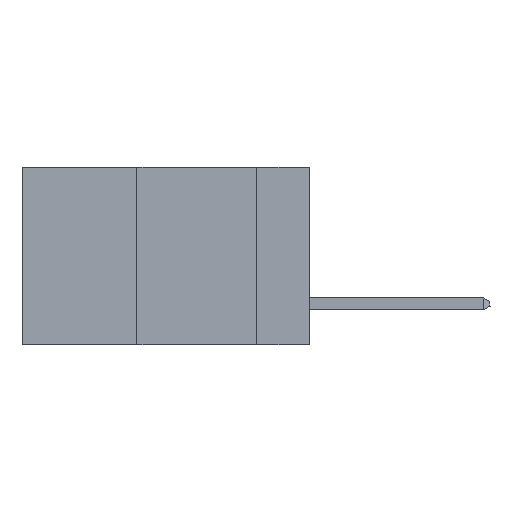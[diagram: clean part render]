
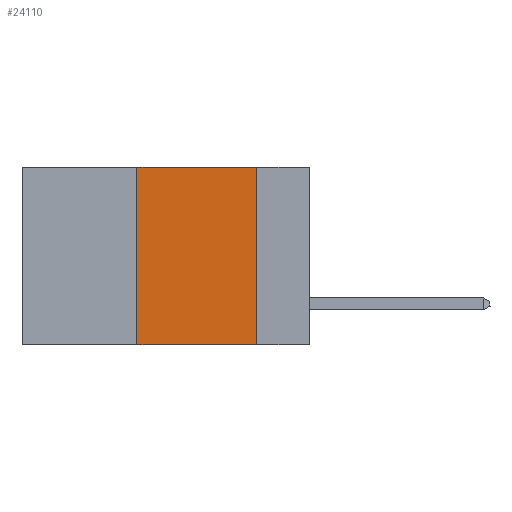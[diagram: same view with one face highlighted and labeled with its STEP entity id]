
A CAD part, left-side view. The second image highlights one B-rep face of the part: STEP entity #24110.
In plain terms, the highlighted planar face has unit normal (-1, 0, 0).
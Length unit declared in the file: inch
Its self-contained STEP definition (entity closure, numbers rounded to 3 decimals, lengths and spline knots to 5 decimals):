
#429 = CARTESIAN_POINT ( 'NONE',  ( 0., 0.6, 0. ) ) ;
#1868 = CARTESIAN_POINT ( 'NONE',  ( 0., 0.11, -0.37 ) ) ;
#2895 = DIRECTION ( 'NONE',  ( 0., 0., -1. ) ) ;
#3239 = ORIENTED_EDGE ( 'NONE', *, *, #12792, .F. ) ;
#3734 = LINE ( 'NONE', #16531, #11338 ) ;
#5599 = PLANE ( 'NONE',  #18371 ) ;
#7148 = DIRECTION ( 'NONE',  ( 0., -1., 0. ) ) ;
#7250 = CARTESIAN_POINT ( 'NONE',  ( 0., 0.11, 0. ) ) ;
#10733 = DIRECTION ( 'NONE',  ( 1., 0., 0. ) ) ;
#11338 = VECTOR ( 'NONE', #7148, 39.37008 ) ;
#11718 = VECTOR ( 'NONE', #18276, 39.37008 ) ;
#12578 = VECTOR ( 'NONE', #23292, 39.37008 ) ;
#12792 = EDGE_CURVE ( 'NONE', #22145, #31823, #23271, .T. ) ;
#13720 = LINE ( 'NONE', #25666, #12578 ) ;
#16531 = CARTESIAN_POINT ( 'NONE',  ( 0., 0.6, -0.37 ) ) ;
#16727 = EDGE_CURVE ( 'NONE', #22037, #23060, #3734, .T. ) ;
#16895 = ORIENTED_EDGE ( 'NONE', *, *, #27657, .F. ) ;
#16928 = FACE_OUTER_BOUND ( 'NONE', #29908, .T. ) ;
#18276 = DIRECTION ( 'NONE',  ( 0., -1., 0. ) ) ;
#18371 = AXIS2_PLACEMENT_3D ( 'NONE', #429, #10733, #2895 ) ;
#19839 = CARTESIAN_POINT ( 'NONE',  ( 0., 0.36, -0.37 ) ) ;
#21968 = LINE ( 'NONE', #7250, #27224 ) ;
#22037 = VERTEX_POINT ( 'NONE', #19839 ) ;
#22043 = DIRECTION ( 'NONE',  ( 0., 0., -1. ) ) ;
#22145 = VERTEX_POINT ( 'NONE', #23518 ) ;
#22545 = CARTESIAN_POINT ( 'NONE',  ( 0., 0.11, 0. ) ) ;
#23060 = VERTEX_POINT ( 'NONE', #1868 ) ;
#23271 = LINE ( 'NONE', #30961, #11718 ) ;
#23292 = DIRECTION ( 'NONE',  ( 0., 0., 1. ) ) ;
#23518 = CARTESIAN_POINT ( 'NONE',  ( 0., 0.36, 0. ) ) ;
#24110 = ADVANCED_FACE ( 'NONE', ( #16928 ), #5599, .F. ) ;
#25666 = CARTESIAN_POINT ( 'NONE',  ( 0., 0.36, 0. ) ) ;
#27224 = VECTOR ( 'NONE', #22043, 39.37008 ) ;
#27657 = EDGE_CURVE ( 'NONE', #22037, #22145, #13720, .T. ) ;
#27969 = ORIENTED_EDGE ( 'NONE', *, *, #29240, .F. ) ;
#29240 = EDGE_CURVE ( 'NONE', #31823, #23060, #21968, .T. ) ;
#29731 = ORIENTED_EDGE ( 'NONE', *, *, #16727, .T. ) ;
#29908 = EDGE_LOOP ( 'NONE', ( #27969, #3239, #16895, #29731 ) ) ;
#30961 = CARTESIAN_POINT ( 'NONE',  ( 0., 0.6, 0. ) ) ;
#31823 = VERTEX_POINT ( 'NONE', #22545 ) ;
